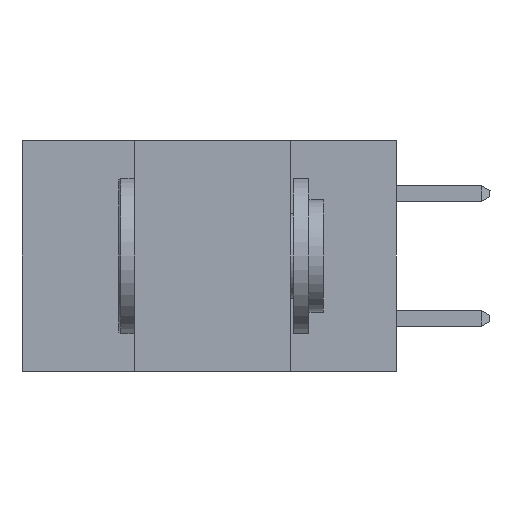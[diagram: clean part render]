
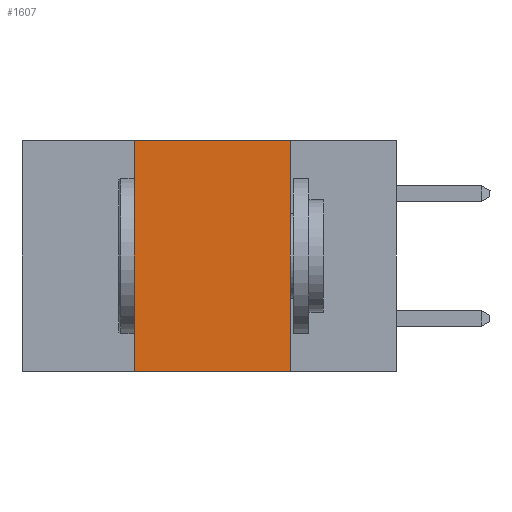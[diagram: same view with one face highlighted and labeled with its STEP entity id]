
A CAD part, left-side view. The second image highlights one B-rep face of the part: STEP entity #1607.
In plain terms, the highlighted planar face has unit normal (-1, 0, 0).
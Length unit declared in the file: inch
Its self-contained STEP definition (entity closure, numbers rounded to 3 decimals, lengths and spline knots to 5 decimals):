
#157 = CARTESIAN_POINT ( 'NONE',  ( 0., 0.6, 0. ) ) ;
#164 = ORIENTED_EDGE ( 'NONE', *, *, #5488, .F. ) ;
#1607 = ADVANCED_FACE ( 'NONE', ( #5083 ), #20297, .F. ) ;
#1662 = LINE ( 'NONE', #7017, #21172 ) ;
#1791 = ORIENTED_EDGE ( 'NONE', *, *, #15756, .T. ) ;
#1860 = CARTESIAN_POINT ( 'NONE',  ( 0., 0.6, 0. ) ) ;
#2844 = DIRECTION ( 'NONE',  ( 0., 0., -1. ) ) ;
#3185 = DIRECTION ( 'NONE',  ( 0., 0., -1. ) ) ;
#3259 = DIRECTION ( 'NONE',  ( 1., 0., 0. ) ) ;
#4314 = VECTOR ( 'NONE', #2844, 39.37008 ) ;
#5083 = FACE_OUTER_BOUND ( 'NONE', #8978, .T. ) ;
#5488 = EDGE_CURVE ( 'NONE', #14882, #24032, #19385, .T. ) ;
#6382 = VECTOR ( 'NONE', #22305, 39.37008 ) ;
#7017 = CARTESIAN_POINT ( 'NONE',  ( 0., 0.6, -0.37 ) ) ;
#8978 = EDGE_LOOP ( 'NONE', ( #164, #16655, #9573, #1791 ) ) ;
#9573 = ORIENTED_EDGE ( 'NONE', *, *, #19512, .F. ) ;
#9648 = CARTESIAN_POINT ( 'NONE',  ( 0., 0.42, -0.37 ) ) ;
#10064 = EDGE_CURVE ( 'NONE', #15790, #14882, #18919, .T. ) ;
#10552 = CARTESIAN_POINT ( 'NONE',  ( 0., 0.17, 0. ) ) ;
#10783 = DIRECTION ( 'NONE',  ( 0., -1., 0. ) ) ;
#10861 = CARTESIAN_POINT ( 'NONE',  ( 0., 0.42, 0. ) ) ;
#11497 = CARTESIAN_POINT ( 'NONE',  ( 0., 0.17, -0.37 ) ) ;
#12012 = CARTESIAN_POINT ( 'NONE',  ( 0., 0.17, 0. ) ) ;
#13955 = AXIS2_PLACEMENT_3D ( 'NONE', #157, #3259, #3185 ) ;
#14641 = LINE ( 'NONE', #20520, #6382 ) ;
#14882 = VERTEX_POINT ( 'NONE', #12012 ) ;
#15756 = EDGE_CURVE ( 'NONE', #20160, #24032, #1662, .T. ) ;
#15790 = VERTEX_POINT ( 'NONE', #10861 ) ;
#16655 = ORIENTED_EDGE ( 'NONE', *, *, #10064, .F. ) ;
#18919 = LINE ( 'NONE', #1860, #23116 ) ;
#19385 = LINE ( 'NONE', #10552, #4314 ) ;
#19512 = EDGE_CURVE ( 'NONE', #20160, #15790, #14641, .T. ) ;
#20160 = VERTEX_POINT ( 'NONE', #9648 ) ;
#20297 = PLANE ( 'NONE',  #13955 ) ;
#20520 = CARTESIAN_POINT ( 'NONE',  ( 0., 0.42, 0. ) ) ;
#20810 = DIRECTION ( 'NONE',  ( 0., -1., 0. ) ) ;
#21172 = VECTOR ( 'NONE', #10783, 39.37008 ) ;
#22305 = DIRECTION ( 'NONE',  ( 0., 0., 1. ) ) ;
#23116 = VECTOR ( 'NONE', #20810, 39.37008 ) ;
#24032 = VERTEX_POINT ( 'NONE', #11497 ) ;
